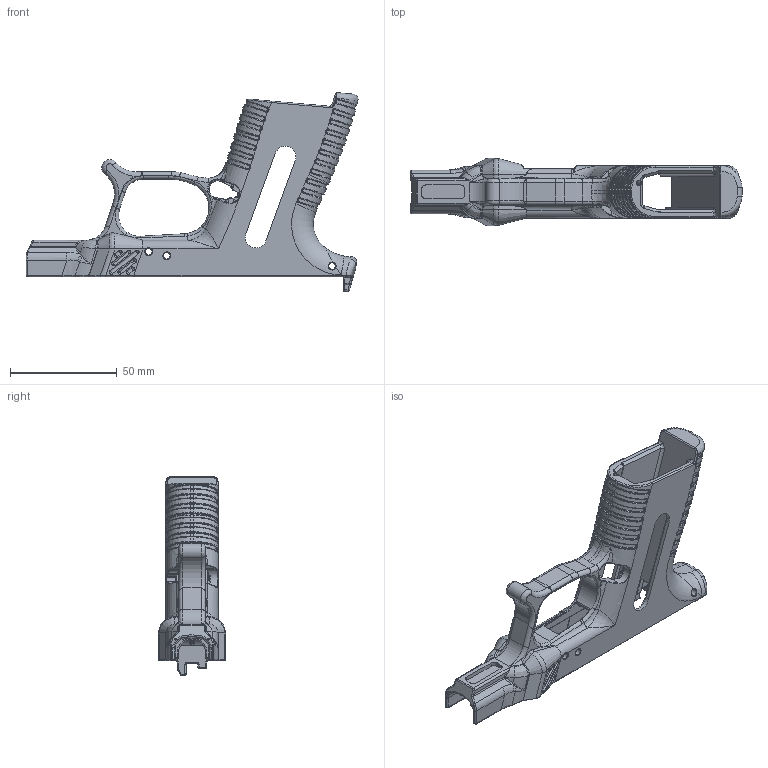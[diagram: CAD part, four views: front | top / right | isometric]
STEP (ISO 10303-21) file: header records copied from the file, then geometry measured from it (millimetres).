
FILE_DESCRIPTION(/* description */ (''),/* implementation_level */ '2;1');
FILE_NAME(/* name */ 'Frame.step',/* time_stamp */ '2020-12-14T21:35:05-05:00',/* author */ (''),/* organization */ (''),/* preprocessor_version */ 'ST-DEVELOPER v18.1',/* originating_system */ 'Autodesk Translation Framework v9.7.1.1290',/* authorisation */ '');
FILE_SCHEMA (('AUTOMOTIVE_DESIGN { 1 0 10303 214 3 1 1 }'));
Products named in the file (1): Frame (1)
Bounding box: 155.35 x 31.41 x 92.92 mm (x, y, z)
Volume: 62347.9 mm3; surface area: 33021.3 mm2
Topology: 1 solids, 1 shells, 1997 faces, 4705 edges, 2648 vertices
Faces by surface type: bspline 845, cylinder 548, torus 286, plane 240, sphere 56, cone 22
Full cylindrical faces by diameter (mm): 1.7 x1, 2 x1, 3.175 x6, 5.715 x1
Entity records: 88113 total; most frequent: CARTESIAN_POINT 45738, ORIENTED_EDGE 9282, DIRECTION 8292, EDGE_CURVE 4641, AXIS2_PLACEMENT_3D 3479, VERTEX_POINT 2647, EDGE_LOOP 2024, FACE_OUTER_BOUND 1996
